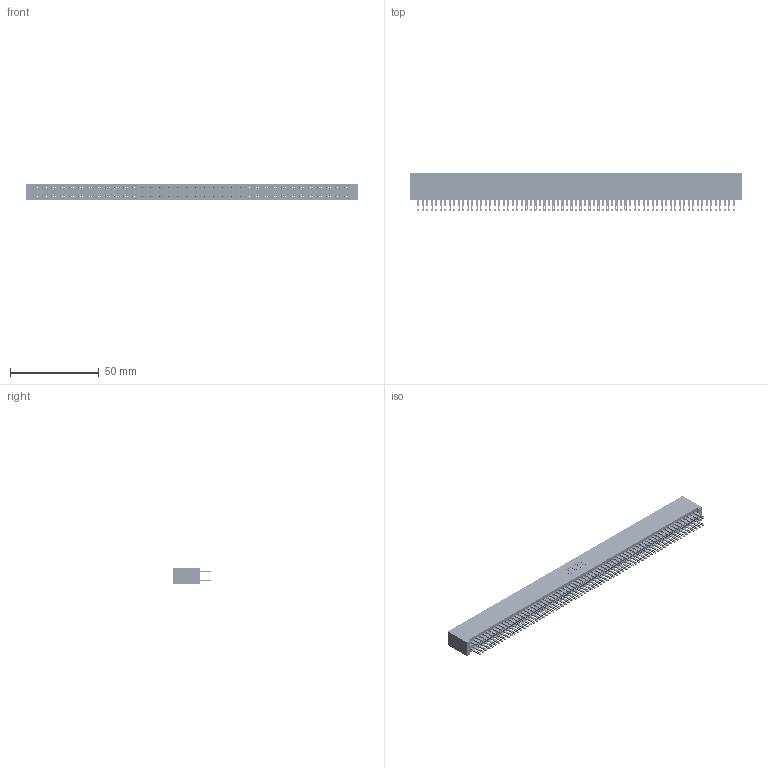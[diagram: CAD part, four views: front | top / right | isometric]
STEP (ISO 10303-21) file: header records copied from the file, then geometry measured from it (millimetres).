
FILE_DESCRIPTION (( 'STEP AP203' ), '1' );
FILE_NAME ('895-142-500-201.STEP', '2020-10-13T19:44:12', ( '' ), ( '' ), 'SwSTEP 2.0', 'SolidWorks 2020', '' );
FILE_SCHEMA (( 'CONFIG_CONTROL_DESIGN' ));
Length unit declared in the file: inch
Products named in the file (3): 845 Part_No Mounting Lugs; 345-292-001_345-293-100; 895-142-500-201
Assembly tree (143 placements, depth 2):
  895-142-500-201
    845 Part_No Mounting Lugs
    345-292-001_345-293-100  x142
Bounding box: 186.94 x 21.51 x 9.4 mm (x, y, z)
Volume: 19479 mm3; surface area: 31106.4 mm2
Topology: 143 solids, 143 shells, 6650 faces, 20339 edges, 13558 vertices
Faces by surface type: plane 3910, cylinder 2740
Entity records: 51457 total; most frequent: CARTESIAN_POINT 8596, ORIENTED_EDGE 8530, DIRECTION 7541, EDGE_CURVE 4265, LINE 3853, VECTOR 3853, VERTEX_POINT 2842, AXIS2_PLACEMENT_3D 1844
